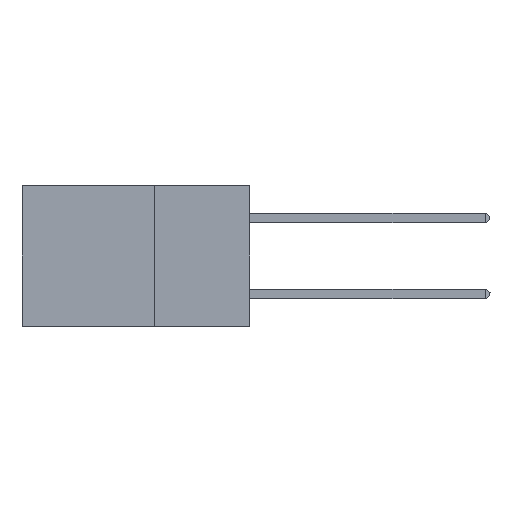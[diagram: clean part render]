
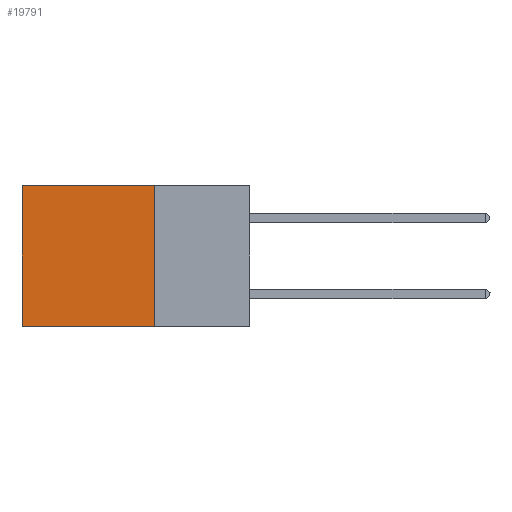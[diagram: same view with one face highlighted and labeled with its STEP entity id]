
A CAD part, left-side view. The second image highlights one B-rep face of the part: STEP entity #19791.
In plain terms, the highlighted planar face has unit normal (-1, 0, 0).
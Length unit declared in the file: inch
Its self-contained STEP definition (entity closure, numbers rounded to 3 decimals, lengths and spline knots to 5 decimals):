
#73 = EDGE_CURVE ( 'NONE', #25497, #13842, #26111, .T. ) ;
#2920 = CARTESIAN_POINT ( 'NONE',  ( 0.2875, 0.25, -0.37 ) ) ;
#3011 = DIRECTION ( 'NONE',  ( 0., 1., 0. ) ) ;
#4979 = AXIS2_PLACEMENT_3D ( 'NONE', #21838, #25634, #11724 ) ;
#7774 = VECTOR ( 'NONE', #43847, 39.37008 ) ;
#8264 = ORIENTED_EDGE ( 'NONE', *, *, #73, .F. ) ;
#11724 = DIRECTION ( 'NONE',  ( 0., 0., -1. ) ) ;
#12496 = CARTESIAN_POINT ( 'NONE',  ( 0.2875, 0.25, 0. ) ) ;
#12681 = CARTESIAN_POINT ( 'NONE',  ( 0.2875, 0.6, -0.37 ) ) ;
#12796 = LINE ( 'NONE', #17104, #33261 ) ;
#13067 = ORIENTED_EDGE ( 'NONE', *, *, #20256, .T. ) ;
#13842 = VERTEX_POINT ( 'NONE', #12681 ) ;
#14290 = LINE ( 'NONE', #24808, #23475 ) ;
#17104 = CARTESIAN_POINT ( 'NONE',  ( 0.2875, 0.25, 0. ) ) ;
#19791 = ADVANCED_FACE ( 'NONE', ( #31140 ), #39303, .F. ) ;
#20256 = EDGE_CURVE ( 'NONE', #32241, #23444, #12796, .T. ) ;
#21838 = CARTESIAN_POINT ( 'NONE',  ( 0.2875, 0.25, 0. ) ) ;
#21904 = CARTESIAN_POINT ( 'NONE',  ( 0.2875, 0.6, 0. ) ) ;
#23444 = VERTEX_POINT ( 'NONE', #32677 ) ;
#23475 = VECTOR ( 'NONE', #27958, 39.37008 ) ;
#24808 = CARTESIAN_POINT ( 'NONE',  ( 0.2875, 0.25, 0. ) ) ;
#24903 = VECTOR ( 'NONE', #28251, 39.37008 ) ;
#25497 = VERTEX_POINT ( 'NONE', #33532 ) ;
#25634 = DIRECTION ( 'NONE',  ( 1., 0., 0. ) ) ;
#25704 = EDGE_CURVE ( 'NONE', #32241, #25497, #14290, .T. ) ;
#26111 = LINE ( 'NONE', #2920, #7774 ) ;
#26683 = ORIENTED_EDGE ( 'NONE', *, *, #43121, .T. ) ;
#27050 = LINE ( 'NONE', #21904, #24903 ) ;
#27958 = DIRECTION ( 'NONE',  ( 0., 0., -1. ) ) ;
#28251 = DIRECTION ( 'NONE',  ( 0., 0., -1. ) ) ;
#31140 = FACE_OUTER_BOUND ( 'NONE', #44317, .T. ) ;
#32241 = VERTEX_POINT ( 'NONE', #12496 ) ;
#32677 = CARTESIAN_POINT ( 'NONE',  ( 0.2875, 0.6, 0. ) ) ;
#33261 = VECTOR ( 'NONE', #3011, 39.37008 ) ;
#33532 = CARTESIAN_POINT ( 'NONE',  ( 0.2875, 0.25, -0.37 ) ) ;
#39303 = PLANE ( 'NONE',  #4979 ) ;
#42254 = ORIENTED_EDGE ( 'NONE', *, *, #25704, .F. ) ;
#43121 = EDGE_CURVE ( 'NONE', #23444, #13842, #27050, .T. ) ;
#43847 = DIRECTION ( 'NONE',  ( 0., 1., 0. ) ) ;
#44317 = EDGE_LOOP ( 'NONE', ( #26683, #8264, #42254, #13067 ) ) ;
